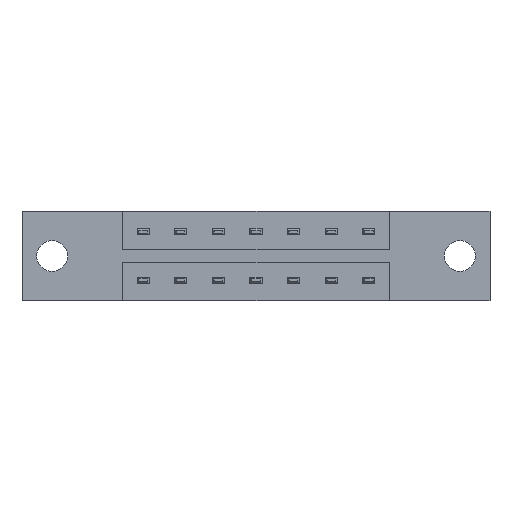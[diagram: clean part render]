
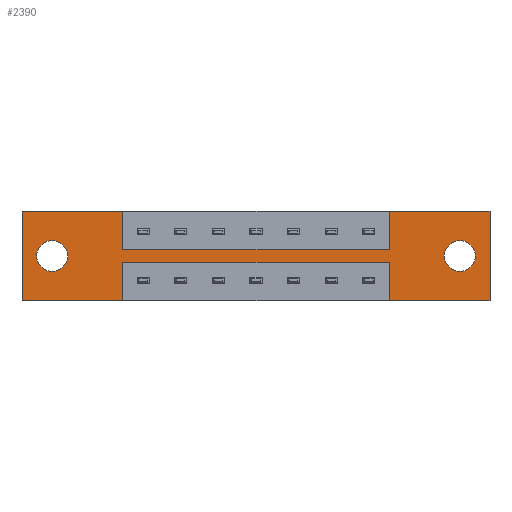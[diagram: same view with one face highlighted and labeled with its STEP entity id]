
A CAD part, front view. The second image highlights one B-rep face of the part: STEP entity #2390.
In plain terms, the highlighted planar face has unit normal (0, -1, 0).
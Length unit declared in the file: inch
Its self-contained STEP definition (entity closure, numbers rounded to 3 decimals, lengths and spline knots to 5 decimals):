
#40 = DIRECTION ( 'NONE',  ( 0., 1., 0. ) ) ;
#205 = VECTOR ( 'NONE', #8649, 39.37008 ) ;
#315 = AXIS2_PLACEMENT_3D ( 'NONE', #8507, #8417, #4362 ) ;
#316 = ORIENTED_EDGE ( 'NONE', *, *, #4823, .T. ) ;
#335 = LINE ( 'NONE', #8546, #2205 ) ;
#366 = CARTESIAN_POINT ( 'NONE',  ( 0., 0., -0.37 ) ) ;
#416 = ORIENTED_EDGE ( 'NONE', *, *, #6371, .F. ) ;
#482 = VECTOR ( 'NONE', #7311, 39.37008 ) ;
#491 = CARTESIAN_POINT ( 'NONE',  ( 0.4175, 0., -0.37 ) ) ;
#556 = AXIS2_PLACEMENT_3D ( 'NONE', #2199, #40, #4328 ) ;
#563 = CIRCLE ( 'NONE', #4744, 0.064 ) ;
#670 = VECTOR ( 'NONE', #4252, 39.37008 ) ;
#693 = VERTEX_POINT ( 'NONE', #6548 ) ;
#705 = CARTESIAN_POINT ( 'NONE',  ( 0.4175, 0., 0. ) ) ;
#841 = CARTESIAN_POINT ( 'NONE',  ( 1.94, 0., -0.37 ) ) ;
#875 = CARTESIAN_POINT ( 'NONE',  ( 1.815, 0., -0.121 ) ) ;
#954 = VERTEX_POINT ( 'NONE', #5062 ) ;
#989 = VERTEX_POINT ( 'NONE', #8308 ) ;
#1027 = PLANE ( 'NONE',  #5333 ) ;
#1169 = FACE_OUTER_BOUND ( 'NONE', #2388, .T. ) ;
#1178 = VECTOR ( 'NONE', #3941, 39.37008 ) ;
#1327 = LINE ( 'NONE', #4081, #7738 ) ;
#1426 = VECTOR ( 'NONE', #6856, 39.37008 ) ;
#1439 = CARTESIAN_POINT ( 'NONE',  ( 0., 0., 0. ) ) ;
#1462 = EDGE_CURVE ( 'NONE', #1847, #3860, #4471, .T. ) ;
#1485 = CARTESIAN_POINT ( 'NONE',  ( 1.94, 0., 0. ) ) ;
#1492 = EDGE_LOOP ( 'NONE', ( #316, #2592 ) ) ;
#1503 = CIRCLE ( 'NONE', #7393, 0.064 ) ;
#1640 = DIRECTION ( 'NONE',  ( -1., 0., 0. ) ) ;
#1835 = VERTEX_POINT ( 'NONE', #841 ) ;
#1847 = VERTEX_POINT ( 'NONE', #4807 ) ;
#1976 = EDGE_CURVE ( 'NONE', #4859, #6539, #2326, .T. ) ;
#1977 = LINE ( 'NONE', #4599, #205 ) ;
#1978 = CARTESIAN_POINT ( 'NONE',  ( 0.4175, 0., -0.2115 ) ) ;
#2098 = ORIENTED_EDGE ( 'NONE', *, *, #3251, .F. ) ;
#2101 = ORIENTED_EDGE ( 'NONE', *, *, #1462, .F. ) ;
#2120 = LINE ( 'NONE', #1485, #7099 ) ;
#2151 = EDGE_CURVE ( 'NONE', #4188, #7180, #6732, .T. ) ;
#2164 = VERTEX_POINT ( 'NONE', #7428 ) ;
#2199 = CARTESIAN_POINT ( 'NONE',  ( 1.815, 0., -0.185 ) ) ;
#2205 = VECTOR ( 'NONE', #6470, 39.37008 ) ;
#2222 = DIRECTION ( 'NONE',  ( 1., 0., 0. ) ) ;
#2248 = EDGE_CURVE ( 'NONE', #7940, #2456, #8181, .T. ) ;
#2275 = CARTESIAN_POINT ( 'NONE',  ( 1.5225, 0., -0.2115 ) ) ;
#2326 = CIRCLE ( 'NONE', #315, 0.064 ) ;
#2388 = EDGE_LOOP ( 'NONE', ( #2098, #6648, #5885, #5186, #3472, #416, #2581, #8212, #2101, #7611, #3685, #3283 ) ) ;
#2390 = ADVANCED_FACE ( 'NONE', ( #5319, #3881, #1169 ), #1027, .T. ) ;
#2456 = VERTEX_POINT ( 'NONE', #491 ) ;
#2470 = DIRECTION ( 'NONE',  ( 0., 0., 1. ) ) ;
#2581 = ORIENTED_EDGE ( 'NONE', *, *, #5249, .F. ) ;
#2592 = ORIENTED_EDGE ( 'NONE', *, *, #8525, .T. ) ;
#2880 = CARTESIAN_POINT ( 'NONE',  ( 1.5225, 0., 0. ) ) ;
#2998 = DIRECTION ( 'NONE',  ( 0., 0., 1. ) ) ;
#3005 = CARTESIAN_POINT ( 'NONE',  ( 0., 0., -0.37 ) ) ;
#3029 = DIRECTION ( 'NONE',  ( 0., 0., -1. ) ) ;
#3042 = VERTEX_POINT ( 'NONE', #705 ) ;
#3152 = LINE ( 'NONE', #3743, #5986 ) ;
#3251 = EDGE_CURVE ( 'NONE', #954, #7408, #335, .T. ) ;
#3283 = ORIENTED_EDGE ( 'NONE', *, *, #8657, .F. ) ;
#3291 = EDGE_CURVE ( 'NONE', #1835, #954, #4493, .T. ) ;
#3472 = ORIENTED_EDGE ( 'NONE', *, *, #5779, .F. ) ;
#3474 = DIRECTION ( 'NONE',  ( 0., 0., -1. ) ) ;
#3605 = EDGE_CURVE ( 'NONE', #3860, #3042, #6283, .T. ) ;
#3685 = ORIENTED_EDGE ( 'NONE', *, *, #2248, .F. ) ;
#3743 = CARTESIAN_POINT ( 'NONE',  ( 0.4175, 0., -0.1585 ) ) ;
#3746 = DIRECTION ( 'NONE',  ( 0., 0., -1. ) ) ;
#3779 = EDGE_CURVE ( 'NONE', #7180, #1835, #2120, .T. ) ;
#3859 = ORIENTED_EDGE ( 'NONE', *, *, #1976, .T. ) ;
#3860 = VERTEX_POINT ( 'NONE', #1439 ) ;
#3881 = FACE_BOUND ( 'NONE', #1492, .T. ) ;
#3899 = CARTESIAN_POINT ( 'NONE',  ( 0., 0., 0. ) ) ;
#3910 = CARTESIAN_POINT ( 'NONE',  ( 1.94, 0., 0. ) ) ;
#3941 = DIRECTION ( 'NONE',  ( 1., 0., 0. ) ) ;
#3954 = CARTESIAN_POINT ( 'NONE',  ( 1.5225, 0., -0.1585 ) ) ;
#4052 = EDGE_CURVE ( 'NONE', #2456, #1847, #1977, .T. ) ;
#4081 = CARTESIAN_POINT ( 'NONE',  ( 0.4175, 0., -0.2115 ) ) ;
#4188 = VERTEX_POINT ( 'NONE', #2880 ) ;
#4206 = CARTESIAN_POINT ( 'NONE',  ( 0., 0., 0. ) ) ;
#4252 = DIRECTION ( 'NONE',  ( 0., 0., -1. ) ) ;
#4328 = DIRECTION ( 'NONE',  ( 0., 0., -1. ) ) ;
#4362 = DIRECTION ( 'NONE',  ( 0., 0., -1. ) ) ;
#4471 = LINE ( 'NONE', #4507, #7282 ) ;
#4488 = CARTESIAN_POINT ( 'NONE',  ( 0.125, 0., -0.185 ) ) ;
#4493 = LINE ( 'NONE', #3005, #7369 ) ;
#4507 = CARTESIAN_POINT ( 'NONE',  ( 0., 0., 0. ) ) ;
#4599 = CARTESIAN_POINT ( 'NONE',  ( 0., 0., -0.37 ) ) ;
#4744 = AXIS2_PLACEMENT_3D ( 'NONE', #6243, #7567, #6911 ) ;
#4807 = CARTESIAN_POINT ( 'NONE',  ( 0., 0., -0.37 ) ) ;
#4823 = EDGE_CURVE ( 'NONE', #989, #7430, #1503, .T. ) ;
#4859 = VERTEX_POINT ( 'NONE', #6380 ) ;
#5062 = CARTESIAN_POINT ( 'NONE',  ( 1.5225, 0., -0.37 ) ) ;
#5163 = EDGE_LOOP ( 'NONE', ( #6418, #3859 ) ) ;
#5186 = ORIENTED_EDGE ( 'NONE', *, *, #2151, .F. ) ;
#5249 = EDGE_CURVE ( 'NONE', #3042, #693, #3152, .T. ) ;
#5319 = FACE_BOUND ( 'NONE', #5163, .T. ) ;
#5333 = AXIS2_PLACEMENT_3D ( 'NONE', #366, #7237, #3746 ) ;
#5428 = CARTESIAN_POINT ( 'NONE',  ( 0.4175, 0., -0.1585 ) ) ;
#5531 = DIRECTION ( 'NONE',  ( -1., 0., 0. ) ) ;
#5779 = EDGE_CURVE ( 'NONE', #2164, #4188, #6700, .T. ) ;
#5805 = DIRECTION ( 'NONE',  ( 0., 1., 0. ) ) ;
#5885 = ORIENTED_EDGE ( 'NONE', *, *, #3779, .F. ) ;
#5986 = VECTOR ( 'NONE', #3029, 39.37008 ) ;
#6101 = VECTOR ( 'NONE', #2222, 39.37008 ) ;
#6243 = CARTESIAN_POINT ( 'NONE',  ( 0.125, 0., -0.185 ) ) ;
#6283 = LINE ( 'NONE', #4206, #6101 ) ;
#6371 = EDGE_CURVE ( 'NONE', #693, #2164, #8179, .T. ) ;
#6380 = CARTESIAN_POINT ( 'NONE',  ( 1.815, 0., -0.249 ) ) ;
#6418 = ORIENTED_EDGE ( 'NONE', *, *, #8108, .T. ) ;
#6470 = DIRECTION ( 'NONE',  ( 0., 0., 1. ) ) ;
#6539 = VERTEX_POINT ( 'NONE', #875 ) ;
#6548 = CARTESIAN_POINT ( 'NONE',  ( 0.4175, 0., -0.1585 ) ) ;
#6648 = ORIENTED_EDGE ( 'NONE', *, *, #3291, .F. ) ;
#6700 = LINE ( 'NONE', #3954, #482 ) ;
#6732 = LINE ( 'NONE', #3899, #1178 ) ;
#6856 = DIRECTION ( 'NONE',  ( 1., 0., 0. ) ) ;
#6911 = DIRECTION ( 'NONE',  ( 0., 0., 1. ) ) ;
#7099 = VECTOR ( 'NONE', #3474, 39.37008 ) ;
#7180 = VERTEX_POINT ( 'NONE', #3910 ) ;
#7237 = DIRECTION ( 'NONE',  ( 0., -1., 0. ) ) ;
#7282 = VECTOR ( 'NONE', #2470, 39.37008 ) ;
#7311 = DIRECTION ( 'NONE',  ( 0., 0., 1. ) ) ;
#7369 = VECTOR ( 'NONE', #1640, 39.37008 ) ;
#7393 = AXIS2_PLACEMENT_3D ( 'NONE', #4488, #5805, #2998 ) ;
#7408 = VERTEX_POINT ( 'NONE', #2275 ) ;
#7428 = CARTESIAN_POINT ( 'NONE',  ( 1.5225, 0., -0.1585 ) ) ;
#7430 = VERTEX_POINT ( 'NONE', #8506 ) ;
#7567 = DIRECTION ( 'NONE',  ( 0., 1., 0. ) ) ;
#7611 = ORIENTED_EDGE ( 'NONE', *, *, #4052, .F. ) ;
#7738 = VECTOR ( 'NONE', #5531, 39.37008 ) ;
#7771 = CARTESIAN_POINT ( 'NONE',  ( 0.4175, 0., -0.2115 ) ) ;
#7940 = VERTEX_POINT ( 'NONE', #1978 ) ;
#8002 = CIRCLE ( 'NONE', #556, 0.064 ) ;
#8108 = EDGE_CURVE ( 'NONE', #6539, #4859, #8002, .T. ) ;
#8179 = LINE ( 'NONE', #5428, #1426 ) ;
#8181 = LINE ( 'NONE', #7771, #670 ) ;
#8212 = ORIENTED_EDGE ( 'NONE', *, *, #3605, .F. ) ;
#8308 = CARTESIAN_POINT ( 'NONE',  ( 0.125, 0., -0.121 ) ) ;
#8417 = DIRECTION ( 'NONE',  ( 0., 1., 0. ) ) ;
#8506 = CARTESIAN_POINT ( 'NONE',  ( 0.125, 0., -0.249 ) ) ;
#8507 = CARTESIAN_POINT ( 'NONE',  ( 1.815, 0., -0.185 ) ) ;
#8525 = EDGE_CURVE ( 'NONE', #7430, #989, #563, .T. ) ;
#8546 = CARTESIAN_POINT ( 'NONE',  ( 1.5225, 0., -0.2115 ) ) ;
#8649 = DIRECTION ( 'NONE',  ( -1., 0., 0. ) ) ;
#8657 = EDGE_CURVE ( 'NONE', #7408, #7940, #1327, .T. ) ;
